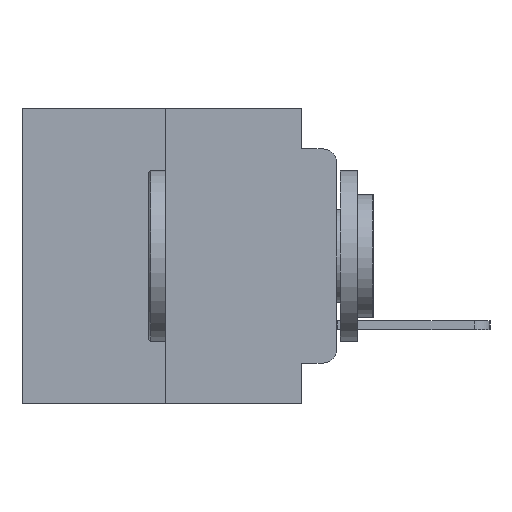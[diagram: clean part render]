
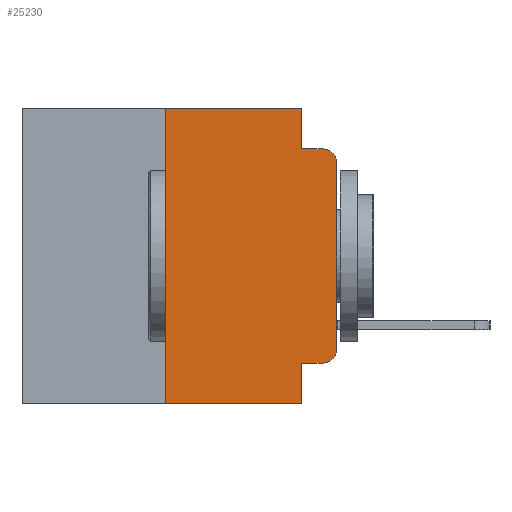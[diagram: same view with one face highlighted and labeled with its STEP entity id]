
A CAD part, left-side view. The second image highlights one B-rep face of the part: STEP entity #25230.
In plain terms, the highlighted planar face has unit normal (-1, 0, 0).
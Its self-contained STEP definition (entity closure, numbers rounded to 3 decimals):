
#422 = DIRECTION ( 'NONE',  ( 0., 0., -1. ) ) ;
#561 = DIRECTION ( 'NONE',  ( -1., 0., 0. ) ) ;
#1292 = VECTOR ( 'NONE', #15696, 1000. ) ;
#1473 = CARTESIAN_POINT ( 'NONE',  ( -75.603, 1.295, -3.975 ) ) ;
#1668 = VERTEX_POINT ( 'NONE', #21327 ) ;
#2245 = VECTOR ( 'NONE', #3823, 1000. ) ;
#3669 = CARTESIAN_POINT ( 'NONE',  ( -75.603, 1.295, 5.486 ) ) ;
#3823 = DIRECTION ( 'NONE',  ( 0., 0., -1. ) ) ;
#3836 = LINE ( 'NONE', #25691, #26595 ) ;
#3959 = LINE ( 'NONE', #15567, #18549 ) ;
#3963 = CARTESIAN_POINT ( 'NONE',  ( -75.603, 0.508, 3.467 ) ) ;
#3996 = ORIENTED_EDGE ( 'NONE', *, *, #9747, .F. ) ;
#4867 = VECTOR ( 'NONE', #11151, 1000. ) ;
#5016 = ORIENTED_EDGE ( 'NONE', *, *, #18725, .F. ) ;
#7502 = CARTESIAN_POINT ( 'NONE',  ( -75.603, 0.508, -3.467 ) ) ;
#7611 = EDGE_CURVE ( 'NONE', #16170, #8559, #28659, .T. ) ;
#8081 = ORIENTED_EDGE ( 'NONE', *, *, #11153, .T. ) ;
#8321 = EDGE_CURVE ( 'NONE', #10726, #17624, #27570, .T. ) ;
#8559 = VERTEX_POINT ( 'NONE', #16359 ) ;
#8602 = DIRECTION ( 'NONE',  ( 0., 0., -1. ) ) ;
#8772 = CARTESIAN_POINT ( 'NONE',  ( -75.603, 6.35, -5.486 ) ) ;
#8789 = CARTESIAN_POINT ( 'NONE',  ( -75.603, 11.684, 5.486 ) ) ;
#8821 = ORIENTED_EDGE ( 'NONE', *, *, #16870, .T. ) ;
#8913 = CARTESIAN_POINT ( 'NONE',  ( -75.603, 0., 5.486 ) ) ;
#9396 = ORIENTED_EDGE ( 'NONE', *, *, #29127, .F. ) ;
#9473 = EDGE_CURVE ( 'NONE', #17624, #8559, #14779, .T. ) ;
#9747 = EDGE_CURVE ( 'NONE', #12597, #22655, #29279, .T. ) ;
#10641 = DIRECTION ( 'NONE',  ( 0., 0., -1. ) ) ;
#10726 = VERTEX_POINT ( 'NONE', #24265 ) ;
#11133 = AXIS2_PLACEMENT_3D ( 'NONE', #7502, #561, #28045 ) ;
#11151 = DIRECTION ( 'NONE',  ( 0., -1., 0. ) ) ;
#11153 = EDGE_CURVE ( 'NONE', #12597, #11202, #14366, .T. ) ;
#11202 = VERTEX_POINT ( 'NONE', #17708 ) ;
#11752 = CARTESIAN_POINT ( 'NONE',  ( -75.603, 1.295, 0. ) ) ;
#12476 = ORIENTED_EDGE ( 'NONE', *, *, #18364, .F. ) ;
#12597 = VERTEX_POINT ( 'NONE', #8772 ) ;
#12750 = ORIENTED_EDGE ( 'NONE', *, *, #8321, .T. ) ;
#13229 = CARTESIAN_POINT ( 'NONE',  ( -75.603, 1.295, 3.975 ) ) ;
#14036 = CARTESIAN_POINT ( 'NONE',  ( -75.603, 0., 3.467 ) ) ;
#14366 = LINE ( 'NONE', #14844, #19683 ) ;
#14491 = DIRECTION ( 'NONE',  ( 0., -1., 0. ) ) ;
#14779 = CIRCLE ( 'NONE', #16360, 0.508 ) ;
#14844 = CARTESIAN_POINT ( 'NONE',  ( -75.603, 11.684, -5.486 ) ) ;
#15567 = CARTESIAN_POINT ( 'NONE',  ( -75.603, 1.295, -3.975 ) ) ;
#15696 = DIRECTION ( 'NONE',  ( 0., 0., 1. ) ) ;
#15781 = DIRECTION ( 'NONE',  ( 0., -1., 0. ) ) ;
#16170 = VERTEX_POINT ( 'NONE', #13229 ) ;
#16359 = CARTESIAN_POINT ( 'NONE',  ( -75.603, 0.508, 3.975 ) ) ;
#16360 = AXIS2_PLACEMENT_3D ( 'NONE', #3963, #24228, #10641 ) ;
#16870 = EDGE_CURVE ( 'NONE', #20919, #1668, #3959, .T. ) ;
#16977 = DIRECTION ( 'NONE',  ( 0., 0., 1. ) ) ;
#17253 = VECTOR ( 'NONE', #16977, 1000. ) ;
#17624 = VERTEX_POINT ( 'NONE', #14036 ) ;
#17708 = CARTESIAN_POINT ( 'NONE',  ( -75.603, 1.295, -5.486 ) ) ;
#18064 = LINE ( 'NONE', #11752, #26558 ) ;
#18364 = EDGE_CURVE ( 'NONE', #22655, #26355, #3836, .T. ) ;
#18549 = VECTOR ( 'NONE', #15781, 1000. ) ;
#18725 = EDGE_CURVE ( 'NONE', #26355, #16170, #18064, .T. ) ;
#19683 = VECTOR ( 'NONE', #24151, 1000. ) ;
#19902 = AXIS2_PLACEMENT_3D ( 'NONE', #8789, #26967, #8602 ) ;
#20571 = ORIENTED_EDGE ( 'NONE', *, *, #23758, .T. ) ;
#20919 = VERTEX_POINT ( 'NONE', #1473 ) ;
#21327 = CARTESIAN_POINT ( 'NONE',  ( -75.603, 0.508, -3.975 ) ) ;
#22218 = PLANE ( 'NONE',  #19902 ) ;
#22655 = VERTEX_POINT ( 'NONE', #26037 ) ;
#23758 = EDGE_CURVE ( 'NONE', #1668, #10726, #28992, .T. ) ;
#24151 = DIRECTION ( 'NONE',  ( 0., -1., 0. ) ) ;
#24228 = DIRECTION ( 'NONE',  ( -1., 0., 0. ) ) ;
#24265 = CARTESIAN_POINT ( 'NONE',  ( -75.603, 0., -3.467 ) ) ;
#25230 = ADVANCED_FACE ( 'NONE', ( #25382 ), #22218, .F. ) ;
#25382 = FACE_OUTER_BOUND ( 'NONE', #29194, .T. ) ;
#25691 = CARTESIAN_POINT ( 'NONE',  ( -75.603, 11.684, 5.486 ) ) ;
#25990 = CARTESIAN_POINT ( 'NONE',  ( -75.603, 6.35, -5.486 ) ) ;
#26037 = CARTESIAN_POINT ( 'NONE',  ( -75.603, 6.35, 5.486 ) ) ;
#26355 = VERTEX_POINT ( 'NONE', #3669 ) ;
#26486 = CARTESIAN_POINT ( 'NONE',  ( -75.603, 1.295, 0. ) ) ;
#26558 = VECTOR ( 'NONE', #422, 1000. ) ;
#26595 = VECTOR ( 'NONE', #14491, 1000. ) ;
#26788 = LINE ( 'NONE', #26486, #2245 ) ;
#26967 = DIRECTION ( 'NONE',  ( 1., 0., 0. ) ) ;
#27321 = ORIENTED_EDGE ( 'NONE', *, *, #9473, .T. ) ;
#27570 = LINE ( 'NONE', #8913, #1292 ) ;
#28045 = DIRECTION ( 'NONE',  ( 0., 0., -1. ) ) ;
#28204 = ORIENTED_EDGE ( 'NONE', *, *, #7611, .F. ) ;
#28659 = LINE ( 'NONE', #29252, #4867 ) ;
#28992 = CIRCLE ( 'NONE', #11133, 0.508 ) ;
#29127 = EDGE_CURVE ( 'NONE', #20919, #11202, #26788, .T. ) ;
#29194 = EDGE_LOOP ( 'NONE', ( #8821, #20571, #12750, #27321, #28204, #5016, #12476, #3996, #8081, #9396 ) ) ;
#29252 = CARTESIAN_POINT ( 'NONE',  ( -75.603, 1.295, 3.975 ) ) ;
#29279 = LINE ( 'NONE', #25990, #17253 ) ;
